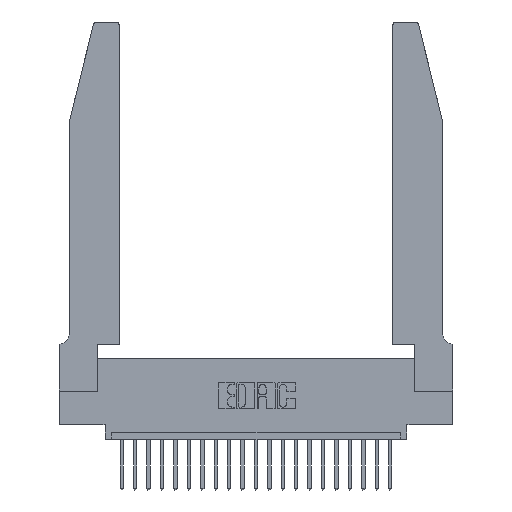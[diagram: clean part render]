
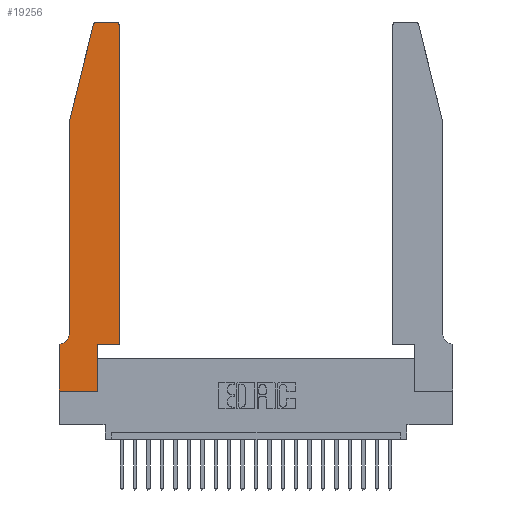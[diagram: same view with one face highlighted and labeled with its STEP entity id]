
A CAD part, top view. The second image highlights one B-rep face of the part: STEP entity #19256.
In plain terms, the highlighted planar face has unit normal (0, 0, 1).
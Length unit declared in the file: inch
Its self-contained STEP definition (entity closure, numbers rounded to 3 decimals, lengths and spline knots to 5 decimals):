
#398 = CARTESIAN_POINT ( 'NONE',  ( 0.0755, 0.42, 0.37 ) ) ;
#689 = DIRECTION ( 'NONE',  ( 0., -1., 0. ) ) ;
#1132 = LINE ( 'NONE', #9378, #16469 ) ;
#1143 = ORIENTED_EDGE ( 'NONE', *, *, #21440, .T. ) ;
#1153 = EDGE_CURVE ( 'NONE', #8503, #17051, #6103, .T. ) ;
#1602 = DIRECTION ( 'NONE',  ( 0., 0., 1. ) ) ;
#1674 = DIRECTION ( 'NONE',  ( 0., 0., -1. ) ) ;
#1713 = CARTESIAN_POINT ( 'NONE',  ( 0.25487, 2.72718, 0.37 ) ) ;
#1886 = EDGE_CURVE ( 'NONE', #11229, #23390, #21966, .T. ) ;
#2336 = VECTOR ( 'NONE', #3259, 39.37008 ) ;
#2404 = DIRECTION ( 'NONE',  ( 1., 0., 0. ) ) ;
#2434 = ORIENTED_EDGE ( 'NONE', *, *, #16169, .T. ) ;
#2814 = CARTESIAN_POINT ( 'NONE',  ( 0., 0., 0.37 ) ) ;
#2863 = LINE ( 'NONE', #11793, #6280 ) ;
#2921 = DIRECTION ( 'NONE',  ( 1., 0., 0. ) ) ;
#3259 = DIRECTION ( 'NONE',  ( 1., 0., 0. ) ) ;
#3640 = ORIENTED_EDGE ( 'NONE', *, *, #4976, .T. ) ;
#3880 = DIRECTION ( 'NONE',  ( -0.239, -0.971, 0. ) ) ;
#4065 = CARTESIAN_POINT ( 'NONE',  ( 0.284, 2.75, 0.37 ) ) ;
#4097 = CARTESIAN_POINT ( 'NONE',  ( 0.4205, 2.72, 0.37 ) ) ;
#4328 = CARTESIAN_POINT ( 'NONE',  ( 0.0755, 2., 0.37 ) ) ;
#4365 = VECTOR ( 'NONE', #16506, 39.37008 ) ;
#4950 = EDGE_CURVE ( 'NONE', #22782, #10909, #1132, .T. ) ;
#4976 = EDGE_CURVE ( 'NONE', #5627, #11229, #12784, .T. ) ;
#5206 = CIRCLE ( 'NONE', #14328, 0.07 ) ;
#5627 = VERTEX_POINT ( 'NONE', #17448 ) ;
#5718 = VERTEX_POINT ( 'NONE', #1713 ) ;
#6103 = LINE ( 'NONE', #7687, #4365 ) ;
#6280 = VECTOR ( 'NONE', #10432, 39.37008 ) ;
#6460 = ORIENTED_EDGE ( 'NONE', *, *, #23113, .T. ) ;
#6831 = AXIS2_PLACEMENT_3D ( 'NONE', #4097, #13294, #2404 ) ;
#7035 = EDGE_CURVE ( 'NONE', #5718, #23094, #9542, .T. ) ;
#7213 = ORIENTED_EDGE ( 'NONE', *, *, #7035, .T. ) ;
#7687 = CARTESIAN_POINT ( 'NONE',  ( 0., 0., 0.37 ) ) ;
#8503 = VERTEX_POINT ( 'NONE', #9640 ) ;
#8717 = CARTESIAN_POINT ( 'NONE',  ( 0., 0., 0.37 ) ) ;
#8886 = CARTESIAN_POINT ( 'NONE',  ( 0.0755, 0.35, 0.37 ) ) ;
#9061 = DIRECTION ( 'NONE',  ( -1., 0., 0. ) ) ;
#9142 = FACE_OUTER_BOUND ( 'NONE', #23318, .T. ) ;
#9378 = CARTESIAN_POINT ( 'NONE',  ( 0.2605, 2.75, 0.37 ) ) ;
#9514 = CARTESIAN_POINT ( 'NONE',  ( 0.4505, 2.72, 0.37 ) ) ;
#9542 = LINE ( 'NONE', #20167, #20647 ) ;
#9640 = CARTESIAN_POINT ( 'NONE',  ( 0., 0.35, 0.37 ) ) ;
#10041 = EDGE_CURVE ( 'NONE', #23094, #19792, #14066, .T. ) ;
#10432 = DIRECTION ( 'NONE',  ( 0., 1., 0. ) ) ;
#10447 = LINE ( 'NONE', #2814, #16701 ) ;
#10596 = CARTESIAN_POINT ( 'NONE',  ( 0.0055, 0.35, 0.37 ) ) ;
#10823 = CARTESIAN_POINT ( 'NONE',  ( 0.0055, 0.42, 0.37 ) ) ;
#10909 = VERTEX_POINT ( 'NONE', #4065 ) ;
#10976 = VECTOR ( 'NONE', #689, 39.37008 ) ;
#10978 = DIRECTION ( 'NONE',  ( -1., 0., 0. ) ) ;
#11001 = EDGE_CURVE ( 'NONE', #10909, #5718, #23153, .T. ) ;
#11229 = VERTEX_POINT ( 'NONE', #11504 ) ;
#11504 = CARTESIAN_POINT ( 'NONE',  ( 0.2865, 0.35, 0.37 ) ) ;
#11756 = EDGE_CURVE ( 'NONE', #16509, #22782, #19707, .T. ) ;
#11793 = CARTESIAN_POINT ( 'NONE',  ( 0.4505, 0.35, 0.37 ) ) ;
#11923 = ORIENTED_EDGE ( 'NONE', *, *, #4950, .T. ) ;
#12262 = DIRECTION ( 'NONE',  ( -1., 0., 0. ) ) ;
#12784 = LINE ( 'NONE', #21496, #20469 ) ;
#13294 = DIRECTION ( 'NONE',  ( 0., 0., 1. ) ) ;
#13881 = CARTESIAN_POINT ( 'NONE',  ( 0.4505, 0.35, 0.37 ) ) ;
#13917 = ORIENTED_EDGE ( 'NONE', *, *, #18806, .T. ) ;
#14066 = LINE ( 'NONE', #16883, #10976 ) ;
#14328 = AXIS2_PLACEMENT_3D ( 'NONE', #10823, #1674, #9061 ) ;
#15599 = AXIS2_PLACEMENT_3D ( 'NONE', #15841, #16488, #20146 ) ;
#15841 = CARTESIAN_POINT ( 'NONE',  ( 0., 0.35, 0.37 ) ) ;
#15943 = ORIENTED_EDGE ( 'NONE', *, *, #10041, .T. ) ;
#16081 = LINE ( 'NONE', #8886, #18915 ) ;
#16169 = EDGE_CURVE ( 'NONE', #23333, #8503, #16081, .T. ) ;
#16469 = VECTOR ( 'NONE', #10978, 39.37008 ) ;
#16488 = DIRECTION ( 'NONE',  ( 0., 0., 1. ) ) ;
#16506 = DIRECTION ( 'NONE',  ( 0., -1., 0. ) ) ;
#16509 = VERTEX_POINT ( 'NONE', #9514 ) ;
#16660 = CARTESIAN_POINT ( 'NONE',  ( 0.4505, 0.35, 0.37 ) ) ;
#16701 = VECTOR ( 'NONE', #19247, 39.37008 ) ;
#16883 = CARTESIAN_POINT ( 'NONE',  ( 0.0755, 2., 0.37 ) ) ;
#17051 = VERTEX_POINT ( 'NONE', #8717 ) ;
#17448 = CARTESIAN_POINT ( 'NONE',  ( 0.2865, 0., 0.37 ) ) ;
#17778 = AXIS2_PLACEMENT_3D ( 'NONE', #23389, #1602, #2921 ) ;
#18771 = ORIENTED_EDGE ( 'NONE', *, *, #1886, .T. ) ;
#18806 = EDGE_CURVE ( 'NONE', #19792, #23333, #5206, .T. ) ;
#18915 = VECTOR ( 'NONE', #12262, 39.37008 ) ;
#19134 = ORIENTED_EDGE ( 'NONE', *, *, #11001, .T. ) ;
#19247 = DIRECTION ( 'NONE',  ( 1., 0., 0. ) ) ;
#19256 = ADVANCED_FACE ( 'NONE', ( #9142 ), #23098, .T. ) ;
#19707 = CIRCLE ( 'NONE', #6831, 0.03 ) ;
#19792 = VERTEX_POINT ( 'NONE', #398 ) ;
#20146 = DIRECTION ( 'NONE',  ( 1., 0., 0. ) ) ;
#20167 = CARTESIAN_POINT ( 'NONE',  ( 0.0755, 2., 0.37 ) ) ;
#20469 = VECTOR ( 'NONE', #23408, 39.37008 ) ;
#20647 = VECTOR ( 'NONE', #3880, 39.37008 ) ;
#21102 = CARTESIAN_POINT ( 'NONE',  ( 0.4205, 2.75, 0.37 ) ) ;
#21440 = EDGE_CURVE ( 'NONE', #17051, #5627, #10447, .T. ) ;
#21496 = CARTESIAN_POINT ( 'NONE',  ( 0.2865, 0.35, 0.37 ) ) ;
#21966 = LINE ( 'NONE', #13881, #2336 ) ;
#22782 = VERTEX_POINT ( 'NONE', #21102 ) ;
#22804 = ORIENTED_EDGE ( 'NONE', *, *, #1153, .T. ) ;
#22985 = ORIENTED_EDGE ( 'NONE', *, *, #11756, .T. ) ;
#23094 = VERTEX_POINT ( 'NONE', #4328 ) ;
#23098 = PLANE ( 'NONE',  #15599 ) ;
#23113 = EDGE_CURVE ( 'NONE', #23390, #16509, #2863, .T. ) ;
#23153 = CIRCLE ( 'NONE', #17778, 0.03 ) ;
#23318 = EDGE_LOOP ( 'NONE', ( #11923, #19134, #7213, #15943, #13917, #2434, #22804, #1143, #3640, #18771, #6460, #22985 ) ) ;
#23333 = VERTEX_POINT ( 'NONE', #10596 ) ;
#23389 = CARTESIAN_POINT ( 'NONE',  ( 0.284, 2.72, 0.37 ) ) ;
#23390 = VERTEX_POINT ( 'NONE', #16660 ) ;
#23408 = DIRECTION ( 'NONE',  ( 0., 1., 0. ) ) ;
